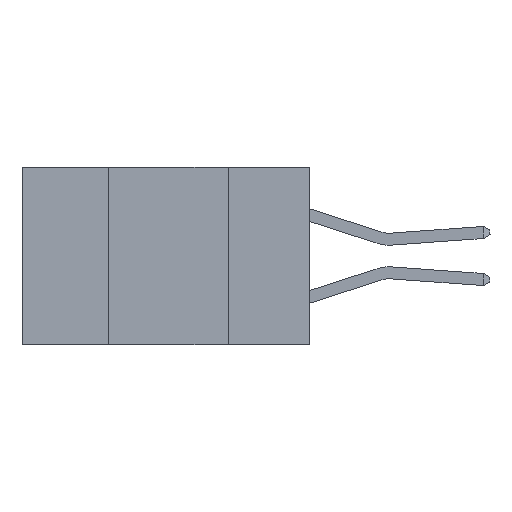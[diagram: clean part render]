
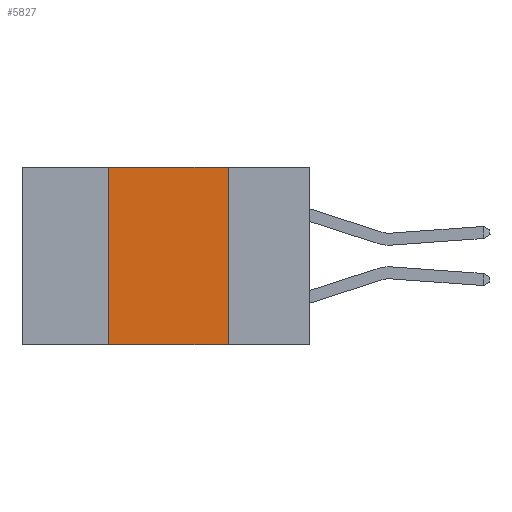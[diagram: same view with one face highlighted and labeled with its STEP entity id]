
A CAD part, left-side view. The second image highlights one B-rep face of the part: STEP entity #5827.
In plain terms, the highlighted planar face has unit normal (-1, 0, 0).
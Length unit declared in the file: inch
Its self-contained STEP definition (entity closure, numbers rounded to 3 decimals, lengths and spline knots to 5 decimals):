
#24 = ORIENTED_EDGE ( 'NONE', *, *, #5924, .F. ) ;
#39 = VERTEX_POINT ( 'NONE', #7392 ) ;
#321 = DIRECTION ( 'NONE',  ( 1., 0., 0. ) ) ;
#364 = LINE ( 'NONE', #8778, #2502 ) ;
#668 = EDGE_CURVE ( 'NONE', #767, #39, #3248, .T. ) ;
#767 = VERTEX_POINT ( 'NONE', #1816 ) ;
#1162 = ORIENTED_EDGE ( 'NONE', *, *, #9008, .T. ) ;
#1331 = CARTESIAN_POINT ( 'NONE',  ( 0., 0.42, -0.37 ) ) ;
#1400 = AXIS2_PLACEMENT_3D ( 'NONE', #7004, #321, #7879 ) ;
#1816 = CARTESIAN_POINT ( 'NONE',  ( 0., 0.17, 0. ) ) ;
#1878 = LINE ( 'NONE', #1331, #3952 ) ;
#2059 = DIRECTION ( 'NONE',  ( 0., -1., 0. ) ) ;
#2340 = VECTOR ( 'NONE', #6216, 39.37008 ) ;
#2502 = VECTOR ( 'NONE', #9382, 39.37008 ) ;
#2823 = CARTESIAN_POINT ( 'NONE',  ( 0., 0.6, -0.37 ) ) ;
#2977 = ORIENTED_EDGE ( 'NONE', *, *, #668, .F. ) ;
#3191 = CARTESIAN_POINT ( 'NONE',  ( 0., 0.17, -0.37 ) ) ;
#3248 = LINE ( 'NONE', #3191, #2340 ) ;
#3952 = VECTOR ( 'NONE', #4926, 39.37008 ) ;
#4631 = FACE_OUTER_BOUND ( 'NONE', #5710, .T. ) ;
#4926 = DIRECTION ( 'NONE',  ( 0., 0., 1. ) ) ;
#5228 = PLANE ( 'NONE',  #1400 ) ;
#5710 = EDGE_LOOP ( 'NONE', ( #2977, #7602, #24, #1162 ) ) ;
#5827 = ADVANCED_FACE ( 'NONE', ( #4631 ), #5228, .F. ) ;
#5924 = EDGE_CURVE ( 'NONE', #7541, #6325, #1878, .T. ) ;
#6048 = EDGE_CURVE ( 'NONE', #6325, #767, #364, .T. ) ;
#6216 = DIRECTION ( 'NONE',  ( 0., 0., -1. ) ) ;
#6227 = VECTOR ( 'NONE', #2059, 39.37008 ) ;
#6325 = VERTEX_POINT ( 'NONE', #9522 ) ;
#6616 = LINE ( 'NONE', #2823, #6227 ) ;
#7004 = CARTESIAN_POINT ( 'NONE',  ( 0., 0.6, 0. ) ) ;
#7392 = CARTESIAN_POINT ( 'NONE',  ( 0., 0.17, -0.37 ) ) ;
#7472 = CARTESIAN_POINT ( 'NONE',  ( 0., 0.42, -0.37 ) ) ;
#7541 = VERTEX_POINT ( 'NONE', #7472 ) ;
#7602 = ORIENTED_EDGE ( 'NONE', *, *, #6048, .F. ) ;
#7879 = DIRECTION ( 'NONE',  ( 0., 0., -1. ) ) ;
#8778 = CARTESIAN_POINT ( 'NONE',  ( 0., 0.6, 0. ) ) ;
#9008 = EDGE_CURVE ( 'NONE', #7541, #39, #6616, .T. ) ;
#9382 = DIRECTION ( 'NONE',  ( 0., -1., 0. ) ) ;
#9522 = CARTESIAN_POINT ( 'NONE',  ( 0., 0.42, 0. ) ) ;
